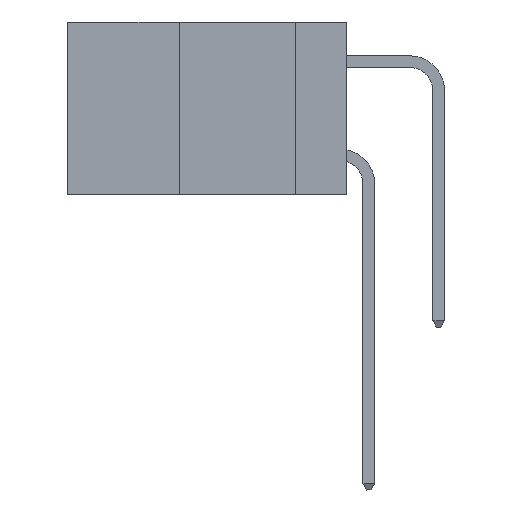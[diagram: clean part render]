
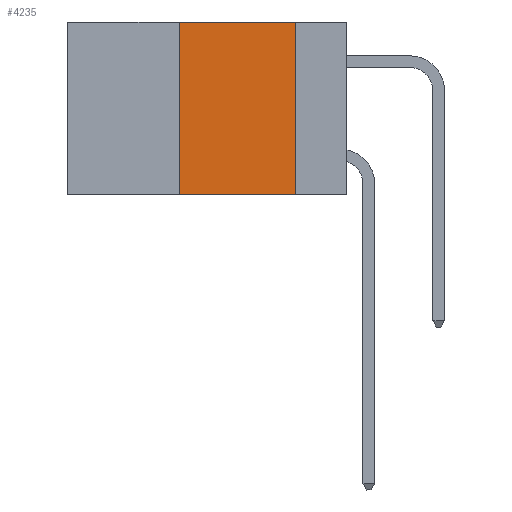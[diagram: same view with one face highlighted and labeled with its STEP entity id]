
A CAD part, left-side view. The second image highlights one B-rep face of the part: STEP entity #4235.
In plain terms, the highlighted planar face has unit normal (-1, 0, 0).
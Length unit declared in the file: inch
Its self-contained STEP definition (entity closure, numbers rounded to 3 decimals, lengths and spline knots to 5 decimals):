
#499 = CARTESIAN_POINT ( 'NONE',  ( 0., 0.11, -0.37 ) ) ;
#1377 = CARTESIAN_POINT ( 'NONE',  ( 0., 0.6, 0. ) ) ;
#1989 = VECTOR ( 'NONE', #10706, 39.37008 ) ;
#2549 = PLANE ( 'NONE',  #15590 ) ;
#2641 = CARTESIAN_POINT ( 'NONE',  ( 0., 0.36, 0. ) ) ;
#2967 = LINE ( 'NONE', #6188, #10435 ) ;
#3465 = FACE_OUTER_BOUND ( 'NONE', #4162, .T. ) ;
#3892 = DIRECTION ( 'NONE',  ( 1., 0., 0. ) ) ;
#4162 = EDGE_LOOP ( 'NONE', ( #8492, #11616, #13625, #10581 ) ) ;
#4235 = ADVANCED_FACE ( 'NONE', ( #3465 ), #2549, .F. ) ;
#5375 = LINE ( 'NONE', #2641, #1989 ) ;
#6165 = LINE ( 'NONE', #12069, #10274 ) ;
#6188 = CARTESIAN_POINT ( 'NONE',  ( 0., 0.11, 0. ) ) ;
#7378 = LINE ( 'NONE', #8643, #14010 ) ;
#7430 = DIRECTION ( 'NONE',  ( 0., 0., -1. ) ) ;
#8206 = VERTEX_POINT ( 'NONE', #9852 ) ;
#8492 = ORIENTED_EDGE ( 'NONE', *, *, #11077, .F. ) ;
#8643 = CARTESIAN_POINT ( 'NONE',  ( 0., 0.6, 0. ) ) ;
#9852 = CARTESIAN_POINT ( 'NONE',  ( 0., 0.11, 0. ) ) ;
#9868 = EDGE_CURVE ( 'NONE', #12095, #8206, #7378, .T. ) ;
#10274 = VECTOR ( 'NONE', #17189, 39.37008 ) ;
#10435 = VECTOR ( 'NONE', #7430, 39.37008 ) ;
#10581 = ORIENTED_EDGE ( 'NONE', *, *, #14309, .T. ) ;
#10584 = CARTESIAN_POINT ( 'NONE',  ( 0., 0.36, 0. ) ) ;
#10670 = DIRECTION ( 'NONE',  ( 0., 0., -1. ) ) ;
#10706 = DIRECTION ( 'NONE',  ( 0., 0., 1. ) ) ;
#11077 = EDGE_CURVE ( 'NONE', #8206, #12185, #2967, .T. ) ;
#11616 = ORIENTED_EDGE ( 'NONE', *, *, #9868, .F. ) ;
#12069 = CARTESIAN_POINT ( 'NONE',  ( 0., 0.6, -0.37 ) ) ;
#12088 = EDGE_CURVE ( 'NONE', #16830, #12095, #5375, .T. ) ;
#12095 = VERTEX_POINT ( 'NONE', #10584 ) ;
#12185 = VERTEX_POINT ( 'NONE', #499 ) ;
#13625 = ORIENTED_EDGE ( 'NONE', *, *, #12088, .F. ) ;
#14010 = VECTOR ( 'NONE', #15398, 39.37008 ) ;
#14309 = EDGE_CURVE ( 'NONE', #16830, #12185, #6165, .T. ) ;
#15292 = CARTESIAN_POINT ( 'NONE',  ( 0., 0.36, -0.37 ) ) ;
#15398 = DIRECTION ( 'NONE',  ( 0., -1., 0. ) ) ;
#15590 = AXIS2_PLACEMENT_3D ( 'NONE', #1377, #3892, #10670 ) ;
#16830 = VERTEX_POINT ( 'NONE', #15292 ) ;
#17189 = DIRECTION ( 'NONE',  ( 0., -1., 0. ) ) ;
